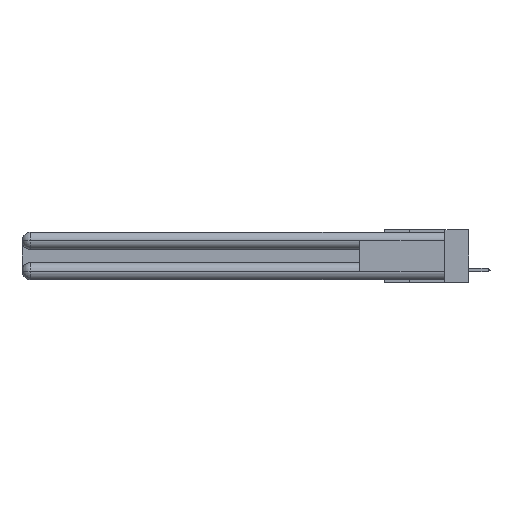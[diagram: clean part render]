
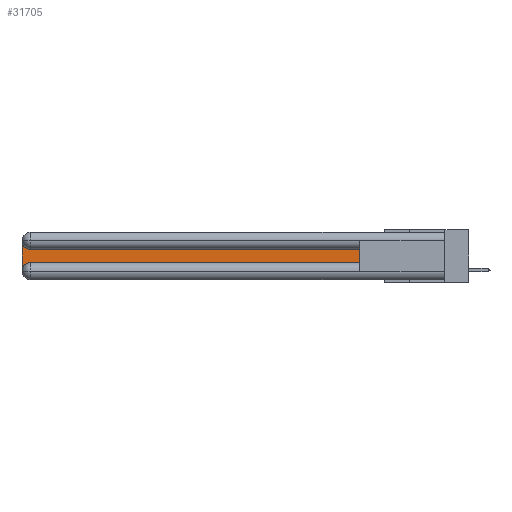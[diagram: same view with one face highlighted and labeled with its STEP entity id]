
A CAD part, left-side view. The second image highlights one B-rep face of the part: STEP entity #31705.
In plain terms, the highlighted planar face has unit normal (-1, 0, 0).
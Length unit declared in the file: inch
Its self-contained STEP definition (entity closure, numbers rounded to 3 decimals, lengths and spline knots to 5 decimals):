
#29 = CARTESIAN_POINT ( 'NONE',  ( 0.075, 2.94, -0.2775 ) ) ;
#218 = CARTESIAN_POINT ( 'NONE',  ( 0.075, 0.6, -0.1225 ) ) ;
#520 = CARTESIAN_POINT ( 'NONE',  ( 0.075, 0.6, -0.1225 ) ) ;
#552 = VERTEX_POINT ( 'NONE', #28724 ) ;
#614 = CIRCLE ( 'NONE', #8177, 0.06 ) ;
#868 = CARTESIAN_POINT ( 'NONE',  ( 0.075, 0.6, -0.2175 ) ) ;
#1368 = LINE ( 'NONE', #868, #28149 ) ;
#1504 = CARTESIAN_POINT ( 'NONE',  ( 0.075, 2.94, -0.2175 ) ) ;
#3473 = DIRECTION ( 'NONE',  ( 0., 0., -1. ) ) ;
#3507 = EDGE_CURVE ( 'NONE', #552, #21698, #30764, .T. ) ;
#3834 = FACE_OUTER_BOUND ( 'NONE', #14320, .T. ) ;
#5387 = DIRECTION ( 'NONE',  ( 0., 0., -1. ) ) ;
#5444 = EDGE_CURVE ( 'NONE', #28411, #32315, #1368, .T. ) ;
#5652 = AXIS2_PLACEMENT_3D ( 'NONE', #16523, #29822, #6203 ) ;
#6203 = DIRECTION ( 'NONE',  ( 0., 0., -1. ) ) ;
#6225 = DIRECTION ( 'NONE',  ( 0., 0., 1. ) ) ;
#7624 = ORIENTED_EDGE ( 'NONE', *, *, #27373, .T. ) ;
#8177 = AXIS2_PLACEMENT_3D ( 'NONE', #8618, #19406, #3473 ) ;
#8259 = CIRCLE ( 'NONE', #23707, 0.06 ) ;
#8618 = CARTESIAN_POINT ( 'NONE',  ( 0.075, 2.94, -0.0625 ) ) ;
#9761 = CARTESIAN_POINT ( 'NONE',  ( 0.075, 0.6, -0.2175 ) ) ;
#11692 = ORIENTED_EDGE ( 'NONE', *, *, #34111, .T. ) ;
#11940 = VECTOR ( 'NONE', #20165, 39.37008 ) ;
#13166 = CARTESIAN_POINT ( 'NONE',  ( 0.075, 2.94, -0.1225 ) ) ;
#13969 = VERTEX_POINT ( 'NONE', #1504 ) ;
#14320 = EDGE_LOOP ( 'NONE', ( #24029, #11692, #25949, #28298, #7624, #21898 ) ) ;
#16523 = CARTESIAN_POINT ( 'NONE',  ( 0.075, 3., -0.1225 ) ) ;
#16530 = VERTEX_POINT ( 'NONE', #13166 ) ;
#16651 = DIRECTION ( 'NONE',  ( 0., 1., 0. ) ) ;
#17371 = LINE ( 'NONE', #30534, #11940 ) ;
#18733 = DIRECTION ( 'NONE',  ( 1., 0., 0. ) ) ;
#19406 = DIRECTION ( 'NONE',  ( 1., 0., 0. ) ) ;
#20165 = DIRECTION ( 'NONE',  ( 0., -1., 0. ) ) ;
#21698 = VERTEX_POINT ( 'NONE', #34004 ) ;
#21898 = ORIENTED_EDGE ( 'NONE', *, *, #5444, .T. ) ;
#23191 = EDGE_CURVE ( 'NONE', #21698, #13969, #8259, .T. ) ;
#23707 = AXIS2_PLACEMENT_3D ( 'NONE', #29, #18733, #5387 ) ;
#24029 = ORIENTED_EDGE ( 'NONE', *, *, #33354, .T. ) ;
#24072 = CARTESIAN_POINT ( 'NONE',  ( 0.075, 3., -0.2175 ) ) ;
#25949 = ORIENTED_EDGE ( 'NONE', *, *, #3507, .T. ) ;
#27186 = PLANE ( 'NONE',  #5652 ) ;
#27373 = EDGE_CURVE ( 'NONE', #13969, #28411, #17371, .T. ) ;
#27892 = VECTOR ( 'NONE', #29614, 39.37008 ) ;
#28149 = VECTOR ( 'NONE', #6225, 39.37008 ) ;
#28298 = ORIENTED_EDGE ( 'NONE', *, *, #23191, .T. ) ;
#28411 = VERTEX_POINT ( 'NONE', #9761 ) ;
#28413 = LINE ( 'NONE', #520, #32164 ) ;
#28724 = CARTESIAN_POINT ( 'NONE',  ( 0.075, 3., -0.0625 ) ) ;
#29614 = DIRECTION ( 'NONE',  ( 0., 0., -1. ) ) ;
#29822 = DIRECTION ( 'NONE',  ( 1., 0., 0. ) ) ;
#30534 = CARTESIAN_POINT ( 'NONE',  ( 0.075, 0.6, -0.2175 ) ) ;
#30764 = LINE ( 'NONE', #24072, #27892 ) ;
#31705 = ADVANCED_FACE ( 'NONE', ( #3834 ), #27186, .F. ) ;
#32164 = VECTOR ( 'NONE', #16651, 39.37008 ) ;
#32315 = VERTEX_POINT ( 'NONE', #218 ) ;
#33354 = EDGE_CURVE ( 'NONE', #32315, #16530, #28413, .T. ) ;
#34004 = CARTESIAN_POINT ( 'NONE',  ( 0.075, 3., -0.2775 ) ) ;
#34111 = EDGE_CURVE ( 'NONE', #16530, #552, #614, .T. ) ;
